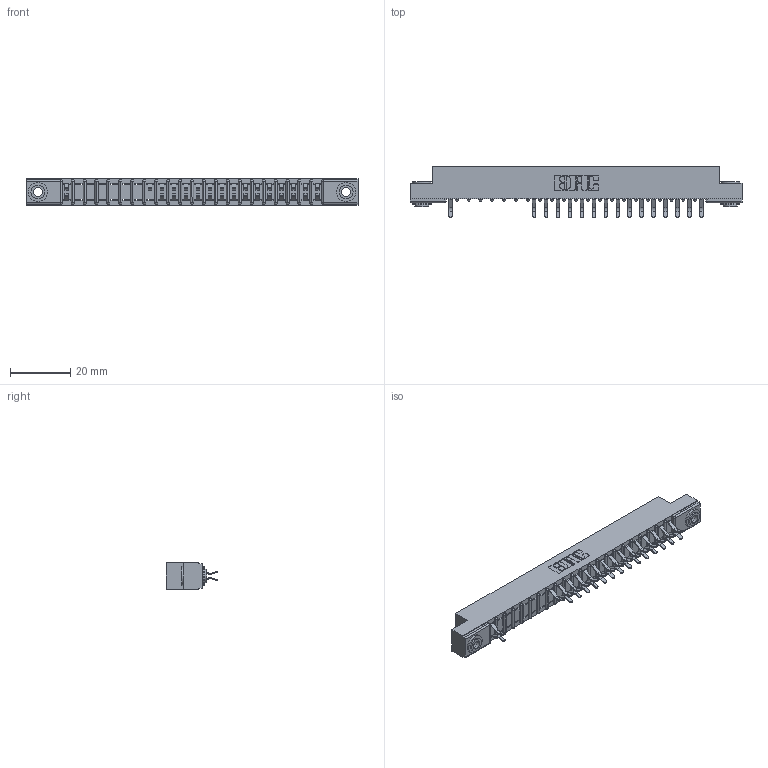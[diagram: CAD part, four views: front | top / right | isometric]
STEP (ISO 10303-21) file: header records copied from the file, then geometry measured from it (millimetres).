
FILE_DESCRIPTION (( 'STEP AP203' ), '1' );
FILE_NAME ('307-044-556-203.STEP', '2018-08-06T02:34:43', ( '' ), ( '' ), 'SwSTEP 2.0', 'SolidWorks 2016', '' );
FILE_SCHEMA (( 'CONFIG_CONTROL_DESIGN' ));
Length unit declared in the file: inch
Products named in the file (4): 307 Part_.156 Dia Mounting Holes; 307-290-001_556; 345-250-002_345-250-002-102; 307-044-556-203
Assembly tree (34 placements, depth 2):
  307-044-556-203
    307 Part_.156 Dia Mounting Holes
    307-290-001_556  x31
    345-250-002_345-250-002-102  x2
Bounding box: 110.19 x 16.97 x 8.71 mm (x, y, z)
Volume: 7034.7 mm3; surface area: 11647.2 mm2
Topology: 34 solids, 34 shells, 1873 faces, 5253 edges, 3394 vertices
Faces by surface type: plane 1195, cylinder 624, sphere 46, cone 8
Entity records: 22783 total; most frequent: CARTESIAN_POINT 3770, ORIENTED_EDGE 3738, DIRECTION 3703, EDGE_CURVE 1869, VECTOR 1417, LINE 1417, VERTEX_POINT 1210, AXIS2_PLACEMENT_3D 1143
